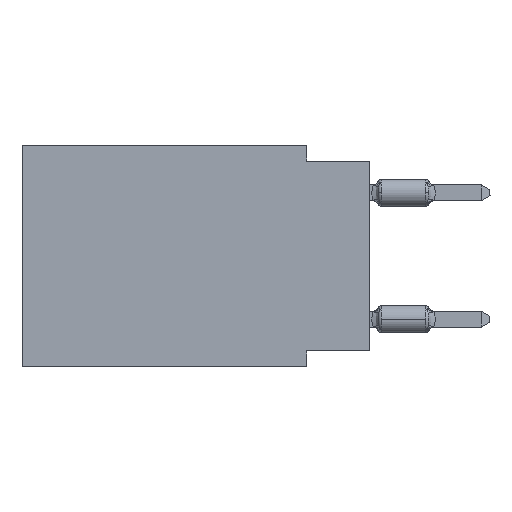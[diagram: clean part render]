
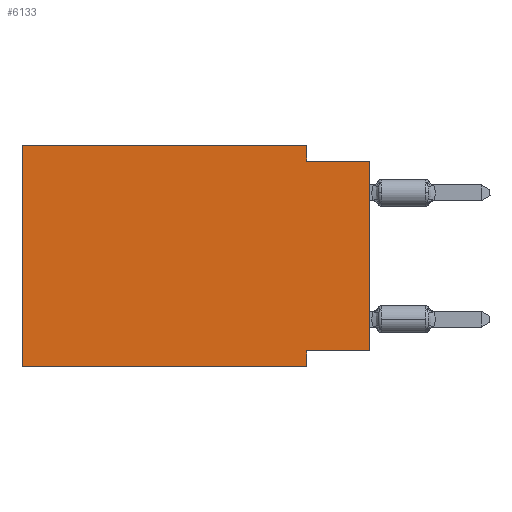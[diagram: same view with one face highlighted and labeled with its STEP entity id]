
A CAD part, left-side view. The second image highlights one B-rep face of the part: STEP entity #6133.
In plain terms, the highlighted planar face has unit normal (-1, 0, 0).
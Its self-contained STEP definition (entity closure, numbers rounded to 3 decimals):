
#53 = FACE_OUTER_BOUND ( 'NONE', #16944, .T. ) ;
#136 = ORIENTED_EDGE ( 'NONE', *, *, #6968, .F. ) ;
#460 = VECTOR ( 'NONE', #10692, 1000. ) ;
#487 = DIRECTION ( 'NONE',  ( 0., -1., 0. ) ) ;
#660 = ORIENTED_EDGE ( 'NONE', *, *, #10062, .F. ) ;
#813 = DIRECTION ( 'NONE',  ( 0., 0., 1. ) ) ;
#1149 = VERTEX_POINT ( 'NONE', #20339 ) ;
#1700 = DIRECTION ( 'NONE',  ( 0., 0., -1. ) ) ;
#2166 = CARTESIAN_POINT ( 'NONE',  ( 0., 0., 0. ) ) ;
#2200 = VECTOR ( 'NONE', #9289, 1000. ) ;
#3225 = CARTESIAN_POINT ( 'NONE',  ( 0., 13.97, -8.89 ) ) ;
#3453 = CARTESIAN_POINT ( 'NONE',  ( 0., 13.97, 0. ) ) ;
#3685 = PLANE ( 'NONE',  #4522 ) ;
#4522 = AXIS2_PLACEMENT_3D ( 'NONE', #3453, #10536, #1700 ) ;
#4568 = LINE ( 'NONE', #20308, #4585 ) ;
#4585 = VECTOR ( 'NONE', #18904, 1000. ) ;
#5041 = CARTESIAN_POINT ( 'NONE',  ( 0., 2.54, -0.635 ) ) ;
#5607 = VERTEX_POINT ( 'NONE', #18072 ) ;
#5996 = CARTESIAN_POINT ( 'NONE',  ( 0., 13.97, -8.89 ) ) ;
#6042 = LINE ( 'NONE', #6392, #18375 ) ;
#6125 = ORIENTED_EDGE ( 'NONE', *, *, #22575, .F. ) ;
#6133 = ADVANCED_FACE ( 'NONE', ( #53 ), #3685, .F. ) ;
#6392 = CARTESIAN_POINT ( 'NONE',  ( 0., 13.97, 0. ) ) ;
#6660 = CARTESIAN_POINT ( 'NONE',  ( 0., 2.54, 0. ) ) ;
#6968 = EDGE_CURVE ( 'NONE', #16403, #1149, #10807, .T. ) ;
#6993 = VERTEX_POINT ( 'NONE', #14783 ) ;
#7243 = EDGE_CURVE ( 'NONE', #12026, #13488, #13382, .T. ) ;
#7821 = LINE ( 'NONE', #10857, #15810 ) ;
#7871 = ORIENTED_EDGE ( 'NONE', *, *, #7243, .T. ) ;
#7914 = CARTESIAN_POINT ( 'NONE',  ( 0., 0., -8.255 ) ) ;
#7923 = EDGE_CURVE ( 'NONE', #10071, #5607, #4568, .T. ) ;
#9289 = DIRECTION ( 'NONE',  ( 0., 0., -1. ) ) ;
#10062 = EDGE_CURVE ( 'NONE', #12026, #6993, #6042, .T. ) ;
#10071 = VERTEX_POINT ( 'NONE', #7914 ) ;
#10208 = VECTOR ( 'NONE', #487, 1000. ) ;
#10536 = DIRECTION ( 'NONE',  ( 1., 0., 0. ) ) ;
#10692 = DIRECTION ( 'NONE',  ( 0., -1., 0. ) ) ;
#10807 = LINE ( 'NONE', #18053, #460 ) ;
#10813 = ORIENTED_EDGE ( 'NONE', *, *, #22553, .F. ) ;
#10857 = CARTESIAN_POINT ( 'NONE',  ( 0., 2.54, 0. ) ) ;
#11146 = CARTESIAN_POINT ( 'NONE',  ( 0., 2.54, -8.89 ) ) ;
#11305 = CARTESIAN_POINT ( 'NONE',  ( 0., 13.97, 0. ) ) ;
#12026 = VERTEX_POINT ( 'NONE', #5996 ) ;
#12252 = CARTESIAN_POINT ( 'NONE',  ( 0., 2.54, -8.89 ) ) ;
#13103 = LINE ( 'NONE', #2166, #20629 ) ;
#13382 = LINE ( 'NONE', #3225, #17602 ) ;
#13488 = VERTEX_POINT ( 'NONE', #12252 ) ;
#14429 = EDGE_CURVE ( 'NONE', #5607, #13488, #23056, .T. ) ;
#14718 = DIRECTION ( 'NONE',  ( 0., 0., -1. ) ) ;
#14783 = CARTESIAN_POINT ( 'NONE',  ( 0., 13.97, 0. ) ) ;
#15314 = ORIENTED_EDGE ( 'NONE', *, *, #22115, .T. ) ;
#15810 = VECTOR ( 'NONE', #14718, 1000. ) ;
#16346 = LINE ( 'NONE', #11305, #10208 ) ;
#16403 = VERTEX_POINT ( 'NONE', #5041 ) ;
#16944 = EDGE_LOOP ( 'NONE', ( #15314, #136, #6125, #10813, #660, #7871, #19489, #18052 ) ) ;
#17602 = VECTOR ( 'NONE', #20477, 1000. ) ;
#18052 = ORIENTED_EDGE ( 'NONE', *, *, #7923, .F. ) ;
#18053 = CARTESIAN_POINT ( 'NONE',  ( 0., 0., -0.635 ) ) ;
#18072 = CARTESIAN_POINT ( 'NONE',  ( 0., 2.54, -8.255 ) ) ;
#18131 = DIRECTION ( 'NONE',  ( 0., 0., 1. ) ) ;
#18375 = VECTOR ( 'NONE', #813, 1000. ) ;
#18904 = DIRECTION ( 'NONE',  ( 0., 1., 0. ) ) ;
#19489 = ORIENTED_EDGE ( 'NONE', *, *, #14429, .F. ) ;
#20308 = CARTESIAN_POINT ( 'NONE',  ( 0., 0., -8.255 ) ) ;
#20339 = CARTESIAN_POINT ( 'NONE',  ( 0., 0., -0.635 ) ) ;
#20477 = DIRECTION ( 'NONE',  ( 0., -1., 0. ) ) ;
#20629 = VECTOR ( 'NONE', #18131, 1000. ) ;
#22115 = EDGE_CURVE ( 'NONE', #10071, #1149, #13103, .T. ) ;
#22231 = VERTEX_POINT ( 'NONE', #6660 ) ;
#22553 = EDGE_CURVE ( 'NONE', #6993, #22231, #16346, .T. ) ;
#22575 = EDGE_CURVE ( 'NONE', #22231, #16403, #7821, .T. ) ;
#23056 = LINE ( 'NONE', #11146, #2200 ) ;
